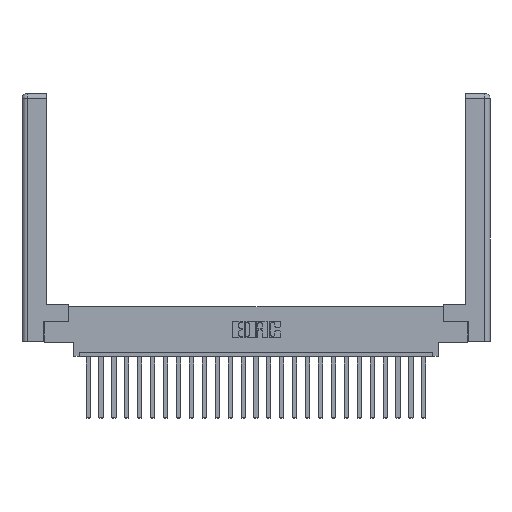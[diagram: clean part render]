
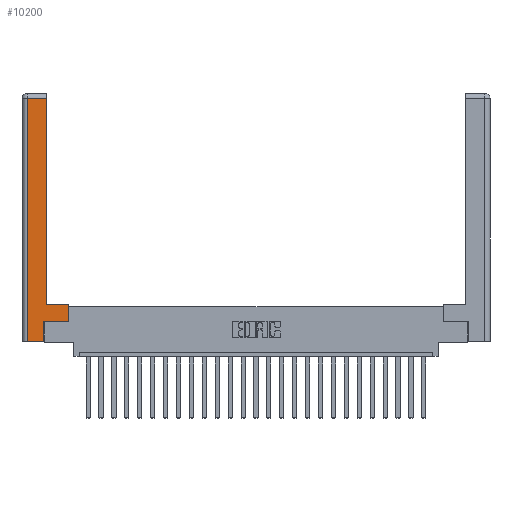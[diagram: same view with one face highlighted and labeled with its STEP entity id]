
A CAD part, top view. The second image highlights one B-rep face of the part: STEP entity #10200.
In plain terms, the highlighted planar face has unit normal (0, 0, 1).
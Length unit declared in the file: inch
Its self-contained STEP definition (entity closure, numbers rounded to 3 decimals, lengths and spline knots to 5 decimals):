
#80 = ORIENTED_EDGE ( 'NONE', *, *, #4072, .T. ) ;
#502 = LINE ( 'NONE', #22327, #9719 ) ;
#977 = CARTESIAN_POINT ( 'NONE',  ( 0.565, 0.245, 0. ) ) ;
#1882 = EDGE_CURVE ( 'NONE', #7752, #12632, #9456, .T. ) ;
#1963 = ORIENTED_EDGE ( 'NONE', *, *, #16058, .T. ) ;
#2637 = LINE ( 'NONE', #977, #17519 ) ;
#2804 = CARTESIAN_POINT ( 'NONE',  ( 0.0615, 2.94, 0. ) ) ;
#3262 = ORIENTED_EDGE ( 'NONE', *, *, #8649, .T. ) ;
#3356 = CARTESIAN_POINT ( 'NONE',  ( 0.265, 0.245, 0. ) ) ;
#4072 = EDGE_CURVE ( 'NONE', #12967, #15945, #11119, .T. ) ;
#5201 = DIRECTION ( 'NONE',  ( 0., 1., 0. ) ) ;
#5225 = EDGE_CURVE ( 'NONE', #22231, #9045, #21228, .T. ) ;
#5712 = CARTESIAN_POINT ( 'NONE',  ( 0.265, 0., 0. ) ) ;
#7684 = VECTOR ( 'NONE', #21848, 39.37008 ) ;
#7752 = VERTEX_POINT ( 'NONE', #19802 ) ;
#8199 = DIRECTION ( 'NONE',  ( 1., 0., 0. ) ) ;
#8517 = FACE_OUTER_BOUND ( 'NONE', #12192, .T. ) ;
#8649 = EDGE_CURVE ( 'NONE', #15945, #22231, #16373, .T. ) ;
#9045 = VERTEX_POINT ( 'NONE', #16277 ) ;
#9354 = ORIENTED_EDGE ( 'NONE', *, *, #1882, .T. ) ;
#9456 = LINE ( 'NONE', #11209, #10615 ) ;
#9719 = VECTOR ( 'NONE', #5201, 39.37008 ) ;
#9884 = VECTOR ( 'NONE', #14906, 39.37008 ) ;
#9986 = ORIENTED_EDGE ( 'NONE', *, *, #16026, .T. ) ;
#10150 = EDGE_CURVE ( 'NONE', #24054, #15868, #502, .T. ) ;
#10200 = ADVANCED_FACE ( 'NONE', ( #8517 ), #14732, .F. ) ;
#10615 = VECTOR ( 'NONE', #20725, 39.37008 ) ;
#11119 = LINE ( 'NONE', #19272, #21566 ) ;
#11209 = CARTESIAN_POINT ( 'NONE',  ( 0.565, 0.45, 0. ) ) ;
#11545 = VECTOR ( 'NONE', #12490, 39.37008 ) ;
#11656 = DIRECTION ( 'NONE',  ( 0., -1., 0. ) ) ;
#12192 = EDGE_LOOP ( 'NONE', ( #15639, #12769, #80, #3262, #12913, #1963, #9354, #9986 ) ) ;
#12490 = DIRECTION ( 'NONE',  ( -1., 0., 0. ) ) ;
#12632 = VERTEX_POINT ( 'NONE', #18158 ) ;
#12769 = ORIENTED_EDGE ( 'NONE', *, *, #23397, .T. ) ;
#12913 = ORIENTED_EDGE ( 'NONE', *, *, #5225, .T. ) ;
#12967 = VERTEX_POINT ( 'NONE', #22560 ) ;
#13459 = CARTESIAN_POINT ( 'NONE',  ( 0.265, 0., 0. ) ) ;
#14732 = PLANE ( 'NONE',  #20211 ) ;
#14906 = DIRECTION ( 'NONE',  ( 0., 1., 0. ) ) ;
#14984 = DIRECTION ( 'NONE',  ( 1., 0., 0. ) ) ;
#15353 = CARTESIAN_POINT ( 'NONE',  ( 0.295, 0.45, 0. ) ) ;
#15639 = ORIENTED_EDGE ( 'NONE', *, *, #10150, .T. ) ;
#15868 = VERTEX_POINT ( 'NONE', #23199 ) ;
#15945 = VERTEX_POINT ( 'NONE', #17775 ) ;
#16026 = EDGE_CURVE ( 'NONE', #12632, #24054, #21085, .T. ) ;
#16058 = EDGE_CURVE ( 'NONE', #9045, #7752, #2637, .T. ) ;
#16124 = CARTESIAN_POINT ( 'NONE',  ( 0.295, 0.45, 0. ) ) ;
#16277 = CARTESIAN_POINT ( 'NONE',  ( 0.265, 0.245, 0. ) ) ;
#16373 = LINE ( 'NONE', #5712, #23215 ) ;
#17519 = VECTOR ( 'NONE', #8199, 39.37008 ) ;
#17775 = CARTESIAN_POINT ( 'NONE',  ( 0.0615, 0., 0. ) ) ;
#18158 = CARTESIAN_POINT ( 'NONE',  ( 0.565, 0.45, 0. ) ) ;
#18579 = CARTESIAN_POINT ( 'NONE',  ( 0., 0., 0. ) ) ;
#18657 = DIRECTION ( 'NONE',  ( -1., 0., 0. ) ) ;
#19272 = CARTESIAN_POINT ( 'NONE',  ( 0.0615, 0., 0. ) ) ;
#19802 = CARTESIAN_POINT ( 'NONE',  ( 0.565, 0.245, 0. ) ) ;
#20211 = AXIS2_PLACEMENT_3D ( 'NONE', #18579, #24279, #18657 ) ;
#20518 = LINE ( 'NONE', #2804, #11545 ) ;
#20725 = DIRECTION ( 'NONE',  ( 0., 1., 0. ) ) ;
#21085 = LINE ( 'NONE', #16124, #7684 ) ;
#21228 = LINE ( 'NONE', #3356, #9884 ) ;
#21566 = VECTOR ( 'NONE', #11656, 39.37008 ) ;
#21848 = DIRECTION ( 'NONE',  ( -1., 0., 0. ) ) ;
#22231 = VERTEX_POINT ( 'NONE', #13459 ) ;
#22327 = CARTESIAN_POINT ( 'NONE',  ( 0.295, 3., 0. ) ) ;
#22560 = CARTESIAN_POINT ( 'NONE',  ( 0.0615, 2.94, 0. ) ) ;
#23199 = CARTESIAN_POINT ( 'NONE',  ( 0.295, 2.94, 0. ) ) ;
#23215 = VECTOR ( 'NONE', #14984, 39.37008 ) ;
#23397 = EDGE_CURVE ( 'NONE', #15868, #12967, #20518, .T. ) ;
#24054 = VERTEX_POINT ( 'NONE', #15353 ) ;
#24279 = DIRECTION ( 'NONE',  ( 0., 0., -1. ) ) ;
